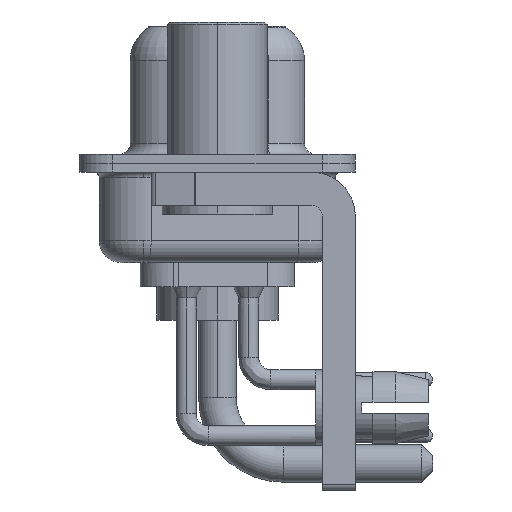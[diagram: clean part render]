
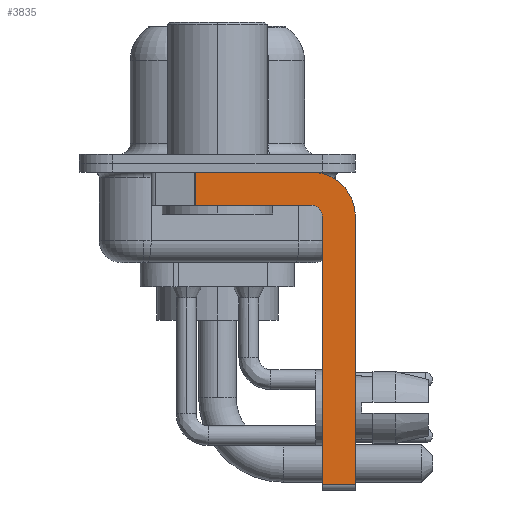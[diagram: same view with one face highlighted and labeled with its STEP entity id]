
A CAD part, left-side view. The second image highlights one B-rep face of the part: STEP entity #3835.
In plain terms, the highlighted planar face has unit normal (-1, 0, 0).
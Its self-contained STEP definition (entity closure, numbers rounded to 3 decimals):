
#10 = VECTOR ( 'NONE', #10611, 1000. ) ;
#441 = LINE ( 'NONE', #12544, #2455 ) ;
#496 = VERTEX_POINT ( 'NONE', #13564 ) ;
#1598 = LINE ( 'NONE', #19377, #18936 ) ;
#1763 = CIRCLE ( 'NONE', #5418, 0.5 ) ;
#1936 = AXIS2_PLACEMENT_3D ( 'NONE', #2862, #20068, #9761 ) ;
#2259 = CARTESIAN_POINT ( 'NONE',  ( -2.9, -4.25, -2.4 ) ) ;
#2455 = VECTOR ( 'NONE', #7138, 1000. ) ;
#2862 = CARTESIAN_POINT ( 'NONE',  ( -2.9, -4.25, -2.4 ) ) ;
#3515 = EDGE_CURVE ( 'NONE', #16416, #496, #1598, .T. ) ;
#3547 = CIRCLE ( 'NONE', #20520, 2. ) ;
#3835 = ADVANCED_FACE ( 'NONE', ( #18220 ), #7693, .F. ) ;
#3839 = VERTEX_POINT ( 'NONE', #6083 ) ;
#4756 = CARTESIAN_POINT ( 'NONE',  ( -2.9, 3., -0.4 ) ) ;
#5200 = LINE ( 'NONE', #4756, #10303 ) ;
#5229 = ORIENTED_EDGE ( 'NONE', *, *, #11008, .F. ) ;
#5418 = AXIS2_PLACEMENT_3D ( 'NONE', #2259, #9269, #9502 ) ;
#5950 = ORIENTED_EDGE ( 'NONE', *, *, #13353, .T. ) ;
#6083 = CARTESIAN_POINT ( 'NONE',  ( -2.9, -4.25, -0.4 ) ) ;
#6307 = ORIENTED_EDGE ( 'NONE', *, *, #13291, .F. ) ;
#7138 = DIRECTION ( 'NONE',  ( 0., 0., 1. ) ) ;
#7343 = EDGE_CURVE ( 'NONE', #21468, #22466, #441, .T. ) ;
#7670 = EDGE_CURVE ( 'NONE', #3839, #12860, #3547, .T. ) ;
#7693 = PLANE ( 'NONE',  #1936 ) ;
#8153 = DIRECTION ( 'NONE',  ( 1., 0., 0. ) ) ;
#8492 = CARTESIAN_POINT ( 'NONE',  ( -2.9, -4.25, -2.4 ) ) ;
#8829 = DIRECTION ( 'NONE',  ( 0., 0., -1. ) ) ;
#8845 = CARTESIAN_POINT ( 'NONE',  ( -2.9, -4.25, -1.9 ) ) ;
#9008 = DIRECTION ( 'NONE',  ( 0., 1., 0. ) ) ;
#9269 = DIRECTION ( 'NONE',  ( -1., 0., 0. ) ) ;
#9502 = DIRECTION ( 'NONE',  ( 0., 0., 1. ) ) ;
#9761 = DIRECTION ( 'NONE',  ( 0., 0., -1. ) ) ;
#10104 = ORIENTED_EDGE ( 'NONE', *, *, #7343, .F. ) ;
#10303 = VECTOR ( 'NONE', #11783, 1000. ) ;
#10336 = LINE ( 'NONE', #13812, #15981 ) ;
#10611 = DIRECTION ( 'NONE',  ( 0., -1., 0. ) ) ;
#10658 = EDGE_CURVE ( 'NONE', #22466, #19283, #1763, .T. ) ;
#11008 = EDGE_CURVE ( 'NONE', #19283, #496, #21151, .T. ) ;
#11501 = VERTEX_POINT ( 'NONE', #15725 ) ;
#11783 = DIRECTION ( 'NONE',  ( 0., -1., 0. ) ) ;
#12544 = CARTESIAN_POINT ( 'NONE',  ( -2.9, -4.75, -14.8 ) ) ;
#12691 = LINE ( 'NONE', #18144, #10 ) ;
#12860 = VERTEX_POINT ( 'NONE', #20824 ) ;
#13291 = EDGE_CURVE ( 'NONE', #16416, #3839, #5200, .T. ) ;
#13353 = EDGE_CURVE ( 'NONE', #21468, #11501, #12691, .T. ) ;
#13564 = CARTESIAN_POINT ( 'NONE',  ( -2.9, 0.978, -1.9 ) ) ;
#13812 = CARTESIAN_POINT ( 'NONE',  ( -2.9, -6.25, -2.4 ) ) ;
#14953 = EDGE_LOOP ( 'NONE', ( #6307, #19823, #5229, #20213, #10104, #5950, #15955, #19849 ) ) ;
#15725 = CARTESIAN_POINT ( 'NONE',  ( -2.9, -6.25, -14.55 ) ) ;
#15955 = ORIENTED_EDGE ( 'NONE', *, *, #22156, .F. ) ;
#15981 = VECTOR ( 'NONE', #8829, 1000. ) ;
#16416 = VERTEX_POINT ( 'NONE', #22491 ) ;
#17029 = CARTESIAN_POINT ( 'NONE',  ( -2.9, -4.75, -2.4 ) ) ;
#17464 = CARTESIAN_POINT ( 'NONE',  ( -2.9, -4.25, -1.9 ) ) ;
#18144 = CARTESIAN_POINT ( 'NONE',  ( -2.9, -4.25, -14.55 ) ) ;
#18220 = FACE_OUTER_BOUND ( 'NONE', #14953, .T. ) ;
#18936 = VECTOR ( 'NONE', #22381, 1000. ) ;
#19283 = VERTEX_POINT ( 'NONE', #8845 ) ;
#19377 = CARTESIAN_POINT ( 'NONE',  ( -2.9, 0.978, -1.9 ) ) ;
#19823 = ORIENTED_EDGE ( 'NONE', *, *, #3515, .T. ) ;
#19849 = ORIENTED_EDGE ( 'NONE', *, *, #7670, .F. ) ;
#20068 = DIRECTION ( 'NONE',  ( 1., 0., 0. ) ) ;
#20213 = ORIENTED_EDGE ( 'NONE', *, *, #10658, .F. ) ;
#20520 = AXIS2_PLACEMENT_3D ( 'NONE', #8492, #8153, #20965 ) ;
#20824 = CARTESIAN_POINT ( 'NONE',  ( -2.9, -6.25, -2.4 ) ) ;
#20965 = DIRECTION ( 'NONE',  ( 0., 0., -1. ) ) ;
#21151 = LINE ( 'NONE', #17464, #22409 ) ;
#21468 = VERTEX_POINT ( 'NONE', #22505 ) ;
#22156 = EDGE_CURVE ( 'NONE', #12860, #11501, #10336, .T. ) ;
#22381 = DIRECTION ( 'NONE',  ( 0., 0., -1. ) ) ;
#22409 = VECTOR ( 'NONE', #9008, 1000. ) ;
#22466 = VERTEX_POINT ( 'NONE', #17029 ) ;
#22491 = CARTESIAN_POINT ( 'NONE',  ( -2.9, 0.978, -0.4 ) ) ;
#22505 = CARTESIAN_POINT ( 'NONE',  ( -2.9, -4.75, -14.55 ) ) ;
